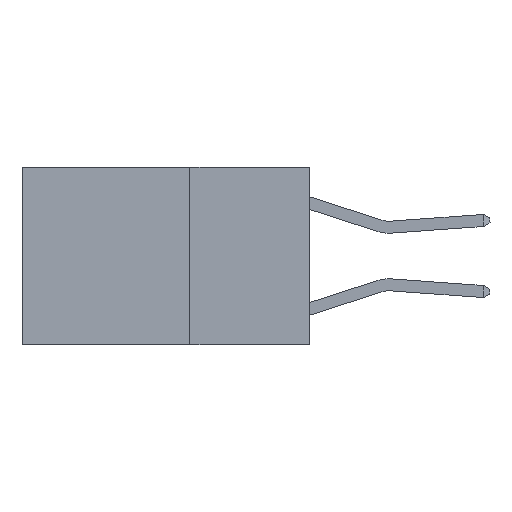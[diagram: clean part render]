
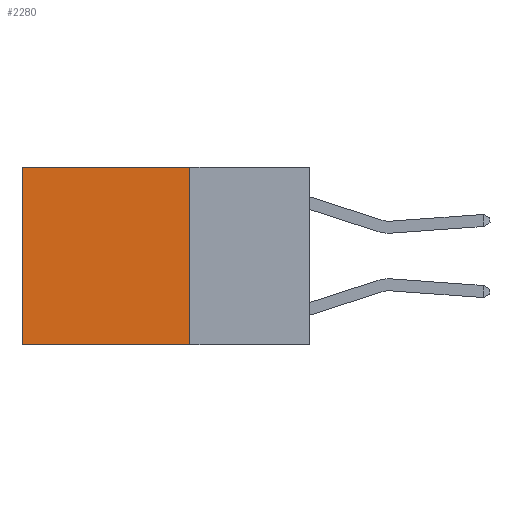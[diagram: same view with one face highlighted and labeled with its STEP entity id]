
A CAD part, left-side view. The second image highlights one B-rep face of the part: STEP entity #2280.
In plain terms, the highlighted planar face has unit normal (-1, 0, 0).
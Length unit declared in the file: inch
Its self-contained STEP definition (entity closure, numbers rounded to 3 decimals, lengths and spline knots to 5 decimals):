
#457 = EDGE_CURVE ( 'NONE', #11262, #8989, #1865, .T. ) ;
#610 = EDGE_CURVE ( 'NONE', #11262, #10630, #4797, .T. ) ;
#1233 = ORIENTED_EDGE ( 'NONE', *, *, #457, .F. ) ;
#1376 = DIRECTION ( 'NONE',  ( 0., 0., -1. ) ) ;
#1865 = LINE ( 'NONE', #2256, #7779 ) ;
#1896 = CARTESIAN_POINT ( 'NONE',  ( 0.2625, 0.25, 0. ) ) ;
#2256 = CARTESIAN_POINT ( 'NONE',  ( 0.2625, 0.25, 0. ) ) ;
#2280 = ADVANCED_FACE ( 'NONE', ( #4902 ), #5447, .F. ) ;
#2815 = DIRECTION ( 'NONE',  ( 0., 1., 0. ) ) ;
#3049 = ORIENTED_EDGE ( 'NONE', *, *, #5332, .F. ) ;
#4744 = ORIENTED_EDGE ( 'NONE', *, *, #8201, .T. ) ;
#4797 = LINE ( 'NONE', #5589, #11422 ) ;
#4902 = FACE_OUTER_BOUND ( 'NONE', #8857, .T. ) ;
#4995 = DIRECTION ( 'NONE',  ( 0., 0., -1. ) ) ;
#5033 = ORIENTED_EDGE ( 'NONE', *, *, #610, .T. ) ;
#5332 = EDGE_CURVE ( 'NONE', #8989, #9220, #7646, .T. ) ;
#5374 = VECTOR ( 'NONE', #2815, 39.37008 ) ;
#5447 = PLANE ( 'NONE',  #8035 ) ;
#5589 = CARTESIAN_POINT ( 'NONE',  ( 0.2625, 0.25, 0. ) ) ;
#5629 = DIRECTION ( 'NONE',  ( 0., 1., 0. ) ) ;
#6603 = CARTESIAN_POINT ( 'NONE',  ( 0.2625, 0.6, 0. ) ) ;
#7646 = LINE ( 'NONE', #8194, #5374 ) ;
#7779 = VECTOR ( 'NONE', #4995, 39.37008 ) ;
#7912 = CARTESIAN_POINT ( 'NONE',  ( 0.2625, 0.6, -0.37 ) ) ;
#8035 = AXIS2_PLACEMENT_3D ( 'NONE', #1896, #10004, #9060 ) ;
#8194 = CARTESIAN_POINT ( 'NONE',  ( 0.2625, 0.25, -0.37 ) ) ;
#8201 = EDGE_CURVE ( 'NONE', #10630, #9220, #9813, .T. ) ;
#8857 = EDGE_LOOP ( 'NONE', ( #4744, #3049, #1233, #5033 ) ) ;
#8975 = VECTOR ( 'NONE', #1376, 39.37008 ) ;
#8989 = VERTEX_POINT ( 'NONE', #9429 ) ;
#9060 = DIRECTION ( 'NONE',  ( 0., 0., -1. ) ) ;
#9220 = VERTEX_POINT ( 'NONE', #7912 ) ;
#9429 = CARTESIAN_POINT ( 'NONE',  ( 0.2625, 0.25, -0.37 ) ) ;
#9813 = LINE ( 'NONE', #6603, #8975 ) ;
#9860 = CARTESIAN_POINT ( 'NONE',  ( 0.2625, 0.25, 0. ) ) ;
#9912 = CARTESIAN_POINT ( 'NONE',  ( 0.2625, 0.6, 0. ) ) ;
#10004 = DIRECTION ( 'NONE',  ( 1., 0., 0. ) ) ;
#10630 = VERTEX_POINT ( 'NONE', #9912 ) ;
#11262 = VERTEX_POINT ( 'NONE', #9860 ) ;
#11422 = VECTOR ( 'NONE', #5629, 39.37008 ) ;
